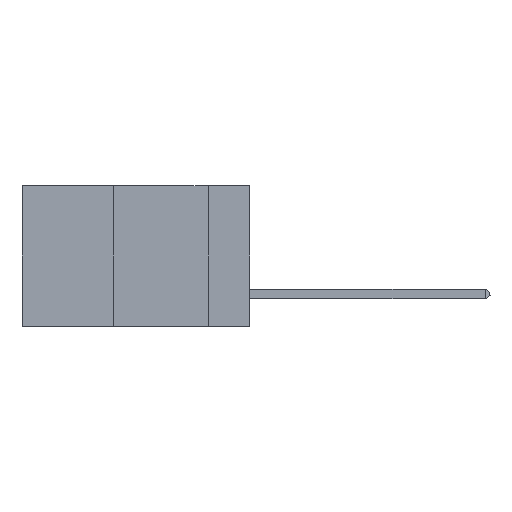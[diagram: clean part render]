
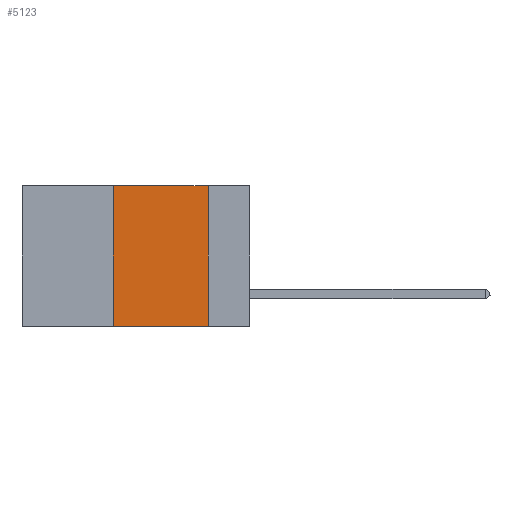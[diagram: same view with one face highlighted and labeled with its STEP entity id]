
A CAD part, left-side view. The second image highlights one B-rep face of the part: STEP entity #5123.
In plain terms, the highlighted planar face has unit normal (-1, 0, 0).
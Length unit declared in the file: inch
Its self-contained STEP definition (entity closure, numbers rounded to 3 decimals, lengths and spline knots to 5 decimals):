
#11 = EDGE_LOOP ( 'NONE', ( #27511, #2572, #22625, #11793 ) ) ;
#1371 = AXIS2_PLACEMENT_3D ( 'NONE', #12213, #11942, #25177 ) ;
#1602 = CARTESIAN_POINT ( 'NONE',  ( 0., 0.6, 0. ) ) ;
#2132 = EDGE_CURVE ( 'NONE', #7370, #9221, #27097, .T. ) ;
#2572 = ORIENTED_EDGE ( 'NONE', *, *, #23198, .F. ) ;
#3069 = DIRECTION ( 'NONE',  ( 0., 0., -1. ) ) ;
#4758 = CARTESIAN_POINT ( 'NONE',  ( 0., 0.36, 0. ) ) ;
#5123 = ADVANCED_FACE ( 'NONE', ( #25329 ), #27338, .F. ) ;
#7370 = VERTEX_POINT ( 'NONE', #23806 ) ;
#7992 = CARTESIAN_POINT ( 'NONE',  ( 0., 0.11, 0. ) ) ;
#9221 = VERTEX_POINT ( 'NONE', #4758 ) ;
#9363 = EDGE_CURVE ( 'NONE', #7370, #12841, #27804, .T. ) ;
#9371 = CARTESIAN_POINT ( 'NONE',  ( 0., 0.36, 0. ) ) ;
#11793 = ORIENTED_EDGE ( 'NONE', *, *, #9363, .T. ) ;
#11942 = DIRECTION ( 'NONE',  ( 1., 0., 0. ) ) ;
#12213 = CARTESIAN_POINT ( 'NONE',  ( 0., 0.6, 0. ) ) ;
#12841 = VERTEX_POINT ( 'NONE', #25447 ) ;
#12857 = VERTEX_POINT ( 'NONE', #7992 ) ;
#14734 = LINE ( 'NONE', #1602, #27849 ) ;
#14968 = CARTESIAN_POINT ( 'NONE',  ( 0., 0.6, -0.37 ) ) ;
#16703 = DIRECTION ( 'NONE',  ( 0., -1., 0. ) ) ;
#17335 = VECTOR ( 'NONE', #3069, 39.37008 ) ;
#17950 = VECTOR ( 'NONE', #18146, 39.37008 ) ;
#18146 = DIRECTION ( 'NONE',  ( 0., 0., 1. ) ) ;
#20807 = CARTESIAN_POINT ( 'NONE',  ( 0., 0.11, 0. ) ) ;
#21220 = DIRECTION ( 'NONE',  ( 0., -1., 0. ) ) ;
#22547 = LINE ( 'NONE', #20807, #17335 ) ;
#22625 = ORIENTED_EDGE ( 'NONE', *, *, #2132, .F. ) ;
#23198 = EDGE_CURVE ( 'NONE', #9221, #12857, #14734, .T. ) ;
#23806 = CARTESIAN_POINT ( 'NONE',  ( 0., 0.36, -0.37 ) ) ;
#24739 = VECTOR ( 'NONE', #16703, 39.37008 ) ;
#25177 = DIRECTION ( 'NONE',  ( 0., 0., -1. ) ) ;
#25329 = FACE_OUTER_BOUND ( 'NONE', #11, .T. ) ;
#25447 = CARTESIAN_POINT ( 'NONE',  ( 0., 0.11, -0.37 ) ) ;
#26919 = EDGE_CURVE ( 'NONE', #12857, #12841, #22547, .T. ) ;
#27097 = LINE ( 'NONE', #9371, #17950 ) ;
#27338 = PLANE ( 'NONE',  #1371 ) ;
#27511 = ORIENTED_EDGE ( 'NONE', *, *, #26919, .F. ) ;
#27804 = LINE ( 'NONE', #14968, #24739 ) ;
#27849 = VECTOR ( 'NONE', #21220, 39.37008 ) ;
